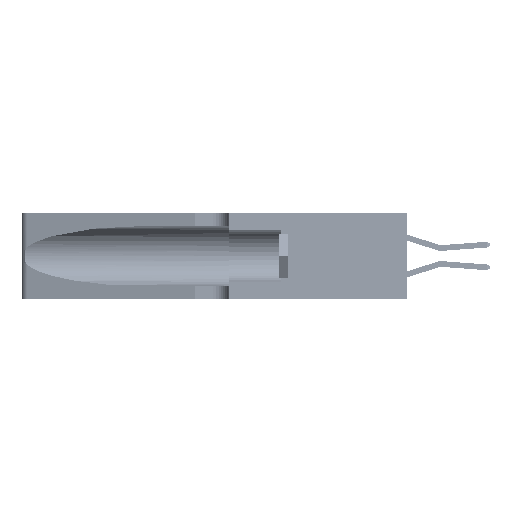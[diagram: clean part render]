
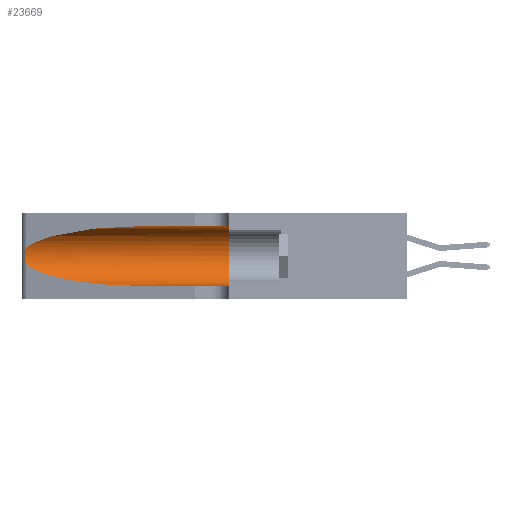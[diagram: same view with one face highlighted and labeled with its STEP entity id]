
A CAD part, left-side view. The second image highlights one B-rep face of the part: STEP entity #23669.
In plain terms, the highlighted cylindrical face has radius 3.308 mm (diameter 6.617 mm), a partial arc.
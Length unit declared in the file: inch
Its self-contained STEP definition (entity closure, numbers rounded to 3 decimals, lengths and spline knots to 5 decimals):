
#1404 =( BOUNDED_CURVE ( )  B_SPLINE_CURVE ( 3, ( #12986, #5408, #24149, #39152 ),
 .UNSPECIFIED., .F., .T. ) 
 B_SPLINE_CURVE_WITH_KNOTS ( ( 4, 4 ),
 ( 3.44316, 4.71239 ),
 .UNSPECIFIED. ) 
 CURVE ( )  GEOMETRIC_REPRESENTATION_ITEM ( )  RATIONAL_B_SPLINE_CURVE ( ( 1., 0.87, 0.87, 1. ) ) 
 REPRESENTATION_ITEM ( '' )  );
#2883 =( BOUNDED_CURVE ( )  B_SPLINE_CURVE ( 3, ( #46569, #20576, #28129, #5613 ),
 .UNSPECIFIED., .F., .F. ) 
 B_SPLINE_CURVE_WITH_KNOTS ( ( 4, 4 ),
 ( 1.5708, 2.84003 ),
 .UNSPECIFIED. ) 
 CURVE ( )  GEOMETRIC_REPRESENTATION_ITEM ( )  RATIONAL_B_SPLINE_CURVE ( ( 1., 0.87, 0.87, 1. ) ) 
 REPRESENTATION_ITEM ( '' )  );
#2986 = VECTOR ( 'NONE', #22855, 39.37008 ) ;
#3609 = DIRECTION ( 'NONE',  ( 0., 1., 0. ) ) ;
#3797 = CARTESIAN_POINT ( 'NONE',  ( 0.25854, 1.2359, 0.20912 ) ) ;
#4424 = VECTOR ( 'NONE', #47137, 39.37008 ) ;
#5408 = CARTESIAN_POINT ( 'NONE',  ( 0.2373, 1.15595, 0.08982 ) ) ;
#5613 = CARTESIAN_POINT ( 'NONE',  ( 0.25487, 1.22718, 0.22369 ) ) ;
#5679 = ORIENTED_EDGE ( 'NONE', *, *, #36101, .F. ) ;
#5748 = VERTEX_POINT ( 'NONE', #31511 ) ;
#7171 = EDGE_CURVE ( 'NONE', #47382, #37137, #1404, .T. ) ;
#7582 = CARTESIAN_POINT ( 'NONE',  ( 0.26075, 1.23896, 0.19203 ) ) ;
#8927 = CIRCLE ( 'NONE', #37472, 0.13025 ) ;
#11395 = CARTESIAN_POINT ( 'NONE',  ( 0.26017, 1.23833, 0.17102 ) ) ;
#11519 = CARTESIAN_POINT ( 'NONE',  ( 0.1305, 0.35, 0.05475 ) ) ;
#12835 = CARTESIAN_POINT ( 'NONE',  ( 0.1305, 1.61858, 0.185 ) ) ;
#12986 = CARTESIAN_POINT ( 'NONE',  ( 0.25487, 1.22718, 0.14631 ) ) ;
#13044 = LINE ( 'NONE', #23019, #2986 ) ;
#13449 = CARTESIAN_POINT ( 'NONE',  ( 0.25487, 1.22718, 0.14631 ) ) ;
#13581 = ORIENTED_EDGE ( 'NONE', *, *, #48180, .T. ) ;
#15173 = CARTESIAN_POINT ( 'NONE',  ( 0.25789, 1.23486, 0.15765 ) ) ;
#15264 = VERTEX_POINT ( 'NONE', #22945 ) ;
#17497 = ORIENTED_EDGE ( 'NONE', *, *, #38028, .F. ) ;
#18940 = CARTESIAN_POINT ( 'NONE',  ( 0.25555, 1.22993, 0.14849 ) ) ;
#20576 = CARTESIAN_POINT ( 'NONE',  ( 0.18966, 0.96281, 0.31525 ) ) ;
#22554 = ORIENTED_EDGE ( 'NONE', *, *, #7171, .T. ) ;
#22561 = CARTESIAN_POINT ( 'NONE',  ( 0.25487, 1.22718, 0.22369 ) ) ;
#22855 = DIRECTION ( 'NONE',  ( 0., -1., 0. ) ) ;
#22945 = CARTESIAN_POINT ( 'NONE',  ( 0.1305, 0.35, 0.31525 ) ) ;
#23019 = CARTESIAN_POINT ( 'NONE',  ( 0.1305, 1.61858, 0.05475 ) ) ;
#23669 = ADVANCED_FACE ( 'NONE', ( #30876 ), #48175, .F. ) ;
#24007 = DIRECTION ( 'NONE',  ( 0., -1., 0. ) ) ;
#24149 = CARTESIAN_POINT ( 'NONE',  ( 0.18966, 0.96281, 0.05475 ) ) ;
#24924 = CARTESIAN_POINT ( 'NONE',  ( 0.1305, 1.61858, 0.31525 ) ) ;
#26129 = CARTESIAN_POINT ( 'NONE',  ( 0.1305, 0.35, 0.185 ) ) ;
#26316 = CARTESIAN_POINT ( 'NONE',  ( 0.25787, 1.23484, 0.2124 ) ) ;
#28129 = CARTESIAN_POINT ( 'NONE',  ( 0.2373, 1.15595, 0.28018 ) ) ;
#29064 = VERTEX_POINT ( 'NONE', #11519 ) ;
#29912 = DIRECTION ( 'NONE',  ( 0., 0., 1. ) ) ;
#30096 = CARTESIAN_POINT ( 'NONE',  ( 0.26018, 1.23835, 0.19895 ) ) ;
#30735 = CARTESIAN_POINT ( 'NONE',  ( 0.1305, 0.72297, 0.05475 ) ) ;
#30876 = FACE_OUTER_BOUND ( 'NONE', #43113, .T. ) ;
#31511 = CARTESIAN_POINT ( 'NONE',  ( 0.25487, 1.22718, 0.22369 ) ) ;
#32032 = CARTESIAN_POINT ( 'NONE',  ( 0.1305, 0.72297, 0.31525 ) ) ;
#32847 = VERTEX_POINT ( 'NONE', #32032 ) ;
#33831 = CARTESIAN_POINT ( 'NONE',  ( 0.26075, 1.23896, 0.178 ) ) ;
#34362 = LINE ( 'NONE', #24924, #4424 ) ;
#36101 = EDGE_CURVE ( 'NONE', #32847, #15264, #34362, .T. ) ;
#36603 = ORIENTED_EDGE ( 'NONE', *, *, #38143, .T. ) ;
#37137 = VERTEX_POINT ( 'NONE', #30735 ) ;
#37472 = AXIS2_PLACEMENT_3D ( 'NONE', #26129, #3609, #29912 ) ;
#37584 = CARTESIAN_POINT ( 'NONE',  ( 0.25856, 1.23593, 0.16098 ) ) ;
#38028 = EDGE_CURVE ( 'NONE', #15264, #29064, #8927, .T. ) ;
#38127 = AXIS2_PLACEMENT_3D ( 'NONE', #12835, #24007, #46214 ) ;
#38143 = EDGE_CURVE ( 'NONE', #37137, #29064, #13044, .T. ) ;
#39152 = CARTESIAN_POINT ( 'NONE',  ( 0.1305, 0.72297, 0.05475 ) ) ;
#41251 = CARTESIAN_POINT ( 'NONE',  ( 0.25639, 1.23186, 0.15144 ) ) ;
#41734 = ORIENTED_EDGE ( 'NONE', *, *, #45687, .T. ) ;
#42774 = B_SPLINE_CURVE_WITH_KNOTS ( 'NONE', 3,
 ( #22561, #44789, #48357, #26316, #3797, #30096, #7582, #33831, #11395, #37584, #15173, #41251, #18940, #44943 ),
 .UNSPECIFIED., .F., .F.,
 ( 4, 2, 2, 2, 2, 2, 4 ),
 ( 0., 0.00027, 0.00053, 0.00107, 0.0016, 0.00187, 0.00214 ),
 .UNSPECIFIED. ) ;
#43113 = EDGE_LOOP ( 'NONE', ( #41734, #13581, #22554, #36603, #17497, #5679 ) ) ;
#44789 = CARTESIAN_POINT ( 'NONE',  ( 0.25555, 1.22994, 0.2215 ) ) ;
#44943 = CARTESIAN_POINT ( 'NONE',  ( 0.25487, 1.22718, 0.14631 ) ) ;
#45687 = EDGE_CURVE ( 'NONE', #32847, #5748, #2883, .T. ) ;
#46214 = DIRECTION ( 'NONE',  ( 0., 0., -1. ) ) ;
#46569 = CARTESIAN_POINT ( 'NONE',  ( 0.1305, 0.72297, 0.31525 ) ) ;
#47137 = DIRECTION ( 'NONE',  ( 0., -1., 0. ) ) ;
#47382 = VERTEX_POINT ( 'NONE', #13449 ) ;
#48175 = CYLINDRICAL_SURFACE ( 'NONE', #38127, 0.13025 ) ;
#48180 = EDGE_CURVE ( 'NONE', #5748, #47382, #42774, .T. ) ;
#48357 = CARTESIAN_POINT ( 'NONE',  ( 0.25639, 1.23184, 0.21858 ) ) ;
